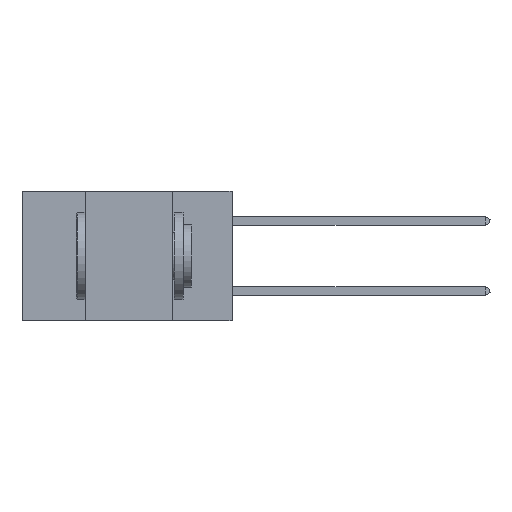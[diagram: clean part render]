
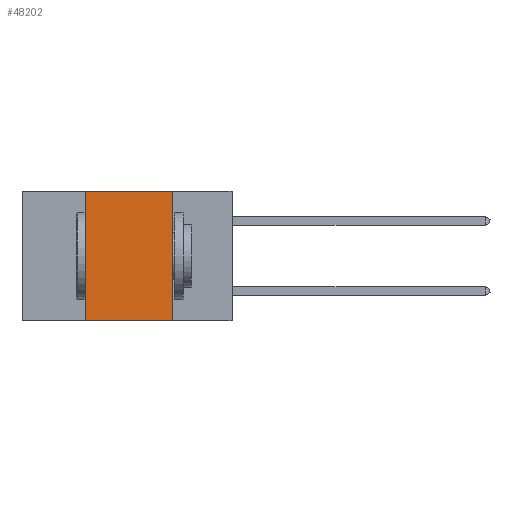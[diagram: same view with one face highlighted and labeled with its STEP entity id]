
A CAD part, left-side view. The second image highlights one B-rep face of the part: STEP entity #48202.
In plain terms, the highlighted planar face has unit normal (-1, 0, 0).
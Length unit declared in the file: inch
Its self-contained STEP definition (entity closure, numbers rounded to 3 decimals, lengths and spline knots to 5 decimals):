
#4652 = VECTOR ( 'NONE', #15723, 39.37008 ) ;
#5308 = CARTESIAN_POINT ( 'NONE',  ( 0., 0.17, -0.37 ) ) ;
#5942 = CARTESIAN_POINT ( 'NONE',  ( 0., 0.17, 0. ) ) ;
#8563 = VERTEX_POINT ( 'NONE', #10471 ) ;
#9804 = PLANE ( 'NONE',  #22066 ) ;
#10248 = EDGE_CURVE ( 'NONE', #8563, #33277, #36918, .T. ) ;
#10471 = CARTESIAN_POINT ( 'NONE',  ( 0., 0.42, -0.37 ) ) ;
#10925 = CARTESIAN_POINT ( 'NONE',  ( 0., 0.17, 0. ) ) ;
#13427 = DIRECTION ( 'NONE',  ( 0., 0., -1. ) ) ;
#13583 = DIRECTION ( 'NONE',  ( 1., 0., 0. ) ) ;
#14637 = CARTESIAN_POINT ( 'NONE',  ( 0., 0.6, 0. ) ) ;
#15723 = DIRECTION ( 'NONE',  ( 0., -1., 0. ) ) ;
#17833 = CARTESIAN_POINT ( 'NONE',  ( 0., 0.6, 0. ) ) ;
#18219 = EDGE_CURVE ( 'NONE', #8563, #44305, #27545, .T. ) ;
#19364 = CARTESIAN_POINT ( 'NONE',  ( 0., 0.42, 0. ) ) ;
#22066 = AXIS2_PLACEMENT_3D ( 'NONE', #17833, #13583, #13427 ) ;
#24500 = DIRECTION ( 'NONE',  ( 0., 0., -1. ) ) ;
#25869 = ORIENTED_EDGE ( 'NONE', *, *, #37940, .F. ) ;
#26652 = LINE ( 'NONE', #5942, #43589 ) ;
#27545 = LINE ( 'NONE', #34969, #4652 ) ;
#28885 = ORIENTED_EDGE ( 'NONE', *, *, #41116, .F. ) ;
#30004 = DIRECTION ( 'NONE',  ( 0., 0., 1. ) ) ;
#30318 = CARTESIAN_POINT ( 'NONE',  ( 0., 0.42, 0. ) ) ;
#30861 = ORIENTED_EDGE ( 'NONE', *, *, #18219, .T. ) ;
#33277 = VERTEX_POINT ( 'NONE', #19364 ) ;
#33433 = DIRECTION ( 'NONE',  ( 0., -1., 0. ) ) ;
#34857 = ORIENTED_EDGE ( 'NONE', *, *, #10248, .F. ) ;
#34969 = CARTESIAN_POINT ( 'NONE',  ( 0., 0.6, -0.37 ) ) ;
#35749 = VECTOR ( 'NONE', #30004, 39.37008 ) ;
#36905 = VERTEX_POINT ( 'NONE', #10925 ) ;
#36918 = LINE ( 'NONE', #30318, #35749 ) ;
#37940 = EDGE_CURVE ( 'NONE', #33277, #36905, #42074, .T. ) ;
#38779 = EDGE_LOOP ( 'NONE', ( #28885, #25869, #34857, #30861 ) ) ;
#39506 = FACE_OUTER_BOUND ( 'NONE', #38779, .T. ) ;
#40947 = VECTOR ( 'NONE', #33433, 39.37008 ) ;
#41116 = EDGE_CURVE ( 'NONE', #36905, #44305, #26652, .T. ) ;
#42074 = LINE ( 'NONE', #14637, #40947 ) ;
#43589 = VECTOR ( 'NONE', #24500, 39.37008 ) ;
#44305 = VERTEX_POINT ( 'NONE', #5308 ) ;
#48202 = ADVANCED_FACE ( 'NONE', ( #39506 ), #9804, .F. ) ;
